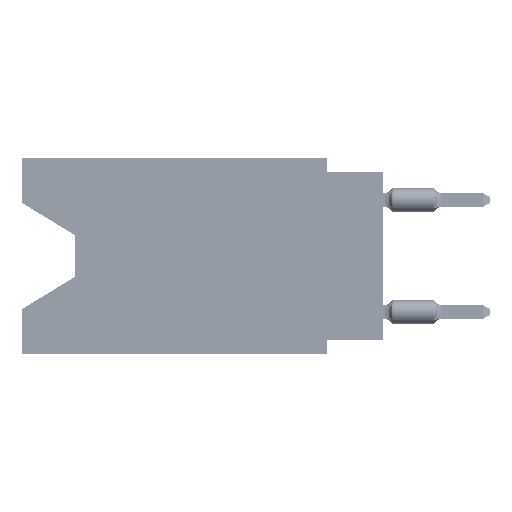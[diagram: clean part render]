
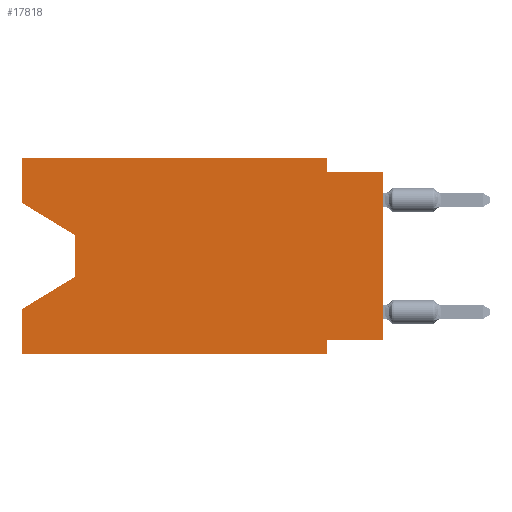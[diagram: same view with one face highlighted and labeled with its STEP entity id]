
A CAD part, left-side view. The second image highlights one B-rep face of the part: STEP entity #17818.
In plain terms, the highlighted planar face has unit normal (-1, 0, 0).
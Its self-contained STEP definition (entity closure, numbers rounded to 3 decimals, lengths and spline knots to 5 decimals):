
#369 = VERTEX_POINT ( 'NONE', #39191 ) ;
#886 = LINE ( 'NONE', #87199, #3611 ) ;
#2932 = CARTESIAN_POINT ( 'NONE',  ( 0., 0.645, 0. ) ) ;
#3611 = VECTOR ( 'NONE', #24710, 39.37008 ) ;
#3846 = EDGE_CURVE ( 'NONE', #369, #61877, #95892, .T. ) ;
#4175 = DIRECTION ( 'NONE',  ( 0., -0.855, -0.519 ) ) ;
#4185 = VECTOR ( 'NONE', #28690, 39.37008 ) ;
#5634 = ORIENTED_EDGE ( 'NONE', *, *, #82824, .F. ) ;
#8033 = LINE ( 'NONE', #78645, #50685 ) ;
#8159 = LINE ( 'NONE', #16301, #43303 ) ;
#11131 = ORIENTED_EDGE ( 'NONE', *, *, #99722, .F. ) ;
#13121 = EDGE_CURVE ( 'NONE', #72424, #53909, #100370, .T. ) ;
#13227 = CARTESIAN_POINT ( 'NONE',  ( 0., 0.1, -0.325 ) ) ;
#15579 = EDGE_LOOP ( 'NONE', ( #20260, #61971, #85714, #86125, #57495, #11131, #67795, #51114, #5634, #78018, #32034, #72724 ) ) ;
#16175 = DIRECTION ( 'NONE',  ( 0., 0., 1. ) ) ;
#16301 = CARTESIAN_POINT ( 'NONE',  ( 0., 0., -0.025 ) ) ;
#17818 = ADVANCED_FACE ( 'NONE', ( #48632 ), #18170, .F. ) ;
#17911 = LINE ( 'NONE', #73275, #41637 ) ;
#18170 = PLANE ( 'NONE',  #48661 ) ;
#20260 = ORIENTED_EDGE ( 'NONE', *, *, #82488, .T. ) ;
#22074 = LINE ( 'NONE', #69293, #4185 ) ;
#22683 = VECTOR ( 'NONE', #86732, 39.37008 ) ;
#22752 = EDGE_CURVE ( 'NONE', #41550, #31722, #63196, .T. ) ;
#23222 = CARTESIAN_POINT ( 'NONE',  ( 0., 0., -0.025 ) ) ;
#24710 = DIRECTION ( 'NONE',  ( 0., 0.855, -0.519 ) ) ;
#24741 = CARTESIAN_POINT ( 'NONE',  ( 0., 0.645, 0. ) ) ;
#25649 = CARTESIAN_POINT ( 'NONE',  ( 0., 0.645, -0.08025 ) ) ;
#27364 = CARTESIAN_POINT ( 'NONE',  ( 0., 0.1, -0.35 ) ) ;
#28690 = DIRECTION ( 'NONE',  ( 0., 0., -1. ) ) ;
#30717 = CARTESIAN_POINT ( 'NONE',  ( 0., 0.645, 0. ) ) ;
#31264 = VERTEX_POINT ( 'NONE', #27364 ) ;
#31722 = VERTEX_POINT ( 'NONE', #62671 ) ;
#32034 = ORIENTED_EDGE ( 'NONE', *, *, #3846, .F. ) ;
#32806 = VERTEX_POINT ( 'NONE', #96971 ) ;
#32838 = VECTOR ( 'NONE', #76645, 39.37008 ) ;
#33909 = DIRECTION ( 'NONE',  ( 0., 0., -1. ) ) ;
#34864 = CARTESIAN_POINT ( 'NONE',  ( 0., 0.645, -0.35 ) ) ;
#37513 = LINE ( 'NONE', #67511, #32838 ) ;
#38393 = VERTEX_POINT ( 'NONE', #56925 ) ;
#39140 = DIRECTION ( 'NONE',  ( 0., -1., 0. ) ) ;
#39191 = CARTESIAN_POINT ( 'NONE',  ( 0., 0.645, 0. ) ) ;
#41550 = VERTEX_POINT ( 'NONE', #47915 ) ;
#41637 = VECTOR ( 'NONE', #4175, 39.37008 ) ;
#42530 = DIRECTION ( 'NONE',  ( 1., 0., 0. ) ) ;
#43303 = VECTOR ( 'NONE', #39140, 39.37008 ) ;
#43469 = VECTOR ( 'NONE', #69831, 39.37008 ) ;
#43889 = CARTESIAN_POINT ( 'NONE',  ( 0., 0.1, 0. ) ) ;
#46169 = VERTEX_POINT ( 'NONE', #25649 ) ;
#46477 = CARTESIAN_POINT ( 'NONE',  ( 0., 0., -0.325 ) ) ;
#46532 = CARTESIAN_POINT ( 'NONE',  ( 0., 0., 0. ) ) ;
#47711 = EDGE_CURVE ( 'NONE', #72424, #84252, #53171, .T. ) ;
#47915 = CARTESIAN_POINT ( 'NONE',  ( 0., 0.645, -0.35 ) ) ;
#48632 = FACE_OUTER_BOUND ( 'NONE', #15579, .T. ) ;
#48661 = AXIS2_PLACEMENT_3D ( 'NONE', #2932, #42530, #33909 ) ;
#50685 = VECTOR ( 'NONE', #16175, 39.37008 ) ;
#51114 = ORIENTED_EDGE ( 'NONE', *, *, #47711, .T. ) ;
#52900 = LINE ( 'NONE', #83873, #93761 ) ;
#53171 = LINE ( 'NONE', #46532, #77056 ) ;
#53909 = VERTEX_POINT ( 'NONE', #13227 ) ;
#56925 = CARTESIAN_POINT ( 'NONE',  ( 0., 0.55, -0.212 ) ) ;
#57254 = CARTESIAN_POINT ( 'NONE',  ( 0., 0.1, -0.025 ) ) ;
#57495 = ORIENTED_EDGE ( 'NONE', *, *, #72119, .T. ) ;
#57708 = VECTOR ( 'NONE', #63834, 39.37008 ) ;
#61877 = VERTEX_POINT ( 'NONE', #43889 ) ;
#61971 = ORIENTED_EDGE ( 'NONE', *, *, #66701, .T. ) ;
#62671 = CARTESIAN_POINT ( 'NONE',  ( 0., 0.645, -0.26975 ) ) ;
#63196 = LINE ( 'NONE', #30717, #43469 ) ;
#63834 = DIRECTION ( 'NONE',  ( 0., -1., 0. ) ) ;
#64320 = LINE ( 'NONE', #34864, #57708 ) ;
#66701 = EDGE_CURVE ( 'NONE', #32806, #38393, #37513, .T. ) ;
#66784 = EDGE_CURVE ( 'NONE', #46169, #369, #8033, .T. ) ;
#67511 = CARTESIAN_POINT ( 'NONE',  ( 0., 0.55, -0.138 ) ) ;
#67795 = ORIENTED_EDGE ( 'NONE', *, *, #13121, .F. ) ;
#67945 = VERTEX_POINT ( 'NONE', #57254 ) ;
#69293 = CARTESIAN_POINT ( 'NONE',  ( 0., 0.1, -0.35 ) ) ;
#69831 = DIRECTION ( 'NONE',  ( 0., 0., 1. ) ) ;
#72119 = EDGE_CURVE ( 'NONE', #41550, #31264, #64320, .T. ) ;
#72424 = VERTEX_POINT ( 'NONE', #46477 ) ;
#72724 = ORIENTED_EDGE ( 'NONE', *, *, #66784, .F. ) ;
#73275 = CARTESIAN_POINT ( 'NONE',  ( 0., 0.645, -0.08025 ) ) ;
#74593 = EDGE_CURVE ( 'NONE', #61877, #67945, #52900, .T. ) ;
#75607 = EDGE_CURVE ( 'NONE', #38393, #31722, #886, .T. ) ;
#76263 = DIRECTION ( 'NONE',  ( 0., 0., -1. ) ) ;
#76645 = DIRECTION ( 'NONE',  ( 0., 0., -1. ) ) ;
#77056 = VECTOR ( 'NONE', #100447, 39.37008 ) ;
#77454 = DIRECTION ( 'NONE',  ( 0., 1., 0. ) ) ;
#78018 = ORIENTED_EDGE ( 'NONE', *, *, #74593, .F. ) ;
#78645 = CARTESIAN_POINT ( 'NONE',  ( 0., 0.645, 0. ) ) ;
#82488 = EDGE_CURVE ( 'NONE', #46169, #32806, #17911, .T. ) ;
#82824 = EDGE_CURVE ( 'NONE', #67945, #84252, #8159, .T. ) ;
#83873 = CARTESIAN_POINT ( 'NONE',  ( 0., 0.1, 0. ) ) ;
#84252 = VERTEX_POINT ( 'NONE', #23222 ) ;
#85714 = ORIENTED_EDGE ( 'NONE', *, *, #75607, .T. ) ;
#86125 = ORIENTED_EDGE ( 'NONE', *, *, #22752, .F. ) ;
#86732 = DIRECTION ( 'NONE',  ( 0., -1., 0. ) ) ;
#87199 = CARTESIAN_POINT ( 'NONE',  ( 0., 0.55, -0.212 ) ) ;
#93761 = VECTOR ( 'NONE', #76263, 39.37008 ) ;
#94302 = VECTOR ( 'NONE', #77454, 39.37008 ) ;
#95892 = LINE ( 'NONE', #24741, #22683 ) ;
#96971 = CARTESIAN_POINT ( 'NONE',  ( 0., 0.55, -0.138 ) ) ;
#99722 = EDGE_CURVE ( 'NONE', #53909, #31264, #22074, .T. ) ;
#99866 = CARTESIAN_POINT ( 'NONE',  ( 0., 0., -0.325 ) ) ;
#100370 = LINE ( 'NONE', #99866, #94302 ) ;
#100447 = DIRECTION ( 'NONE',  ( 0., 0., 1. ) ) ;
